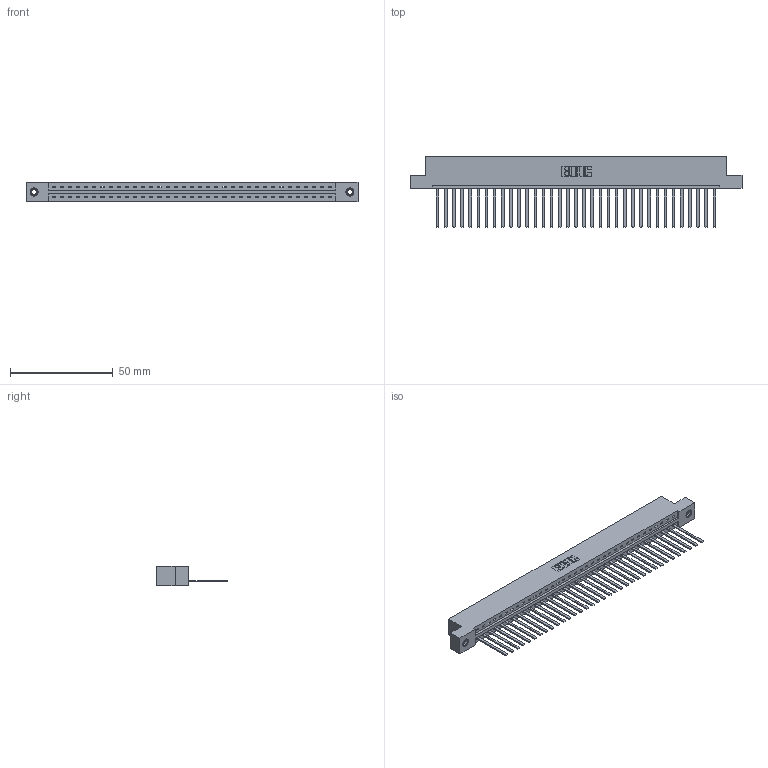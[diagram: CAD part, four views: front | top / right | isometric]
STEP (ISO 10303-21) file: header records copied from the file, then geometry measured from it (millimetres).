
FILE_DESCRIPTION (( 'STEP AP203' ), '1' );
FILE_NAME ('387-035-544-107.STEP', '2018-09-18T22:42:55', ( '' ), ( '' ), 'SwSTEP 2.0', 'SolidWorks 2016', '' );
FILE_SCHEMA (( 'CONFIG_CONTROL_DESIGN' ));
Length unit declared in the file: inch
Products named in the file (4): 337 Part_Flush Mounting Lugs - 0.156 Dia-TI; 345-292-001_345-293-144; 345-250-001_345-250-005-103; 387-035-544-107
Assembly tree (38 placements, depth 2):
  387-035-544-107
    337 Part_Flush Mounting Lugs - 0.156 Dia-TI
    345-292-001_345-293-144  x35
    345-250-001_345-250-005-103  x2
Bounding box: 161.7 x 34.3 x 9.4 mm (x, y, z)
Volume: 17109.9 mm3; surface area: 19016.1 mm2
Topology: 38 solids, 38 shells, 2134 faces, 6397 edges, 4210 vertices
Faces by surface type: plane 1572, cylinder 546, cone 12, torus 4
Entity records: 27924 total; most frequent: CARTESIAN_POINT 4842, ORIENTED_EDGE 4806, DIRECTION 4119, EDGE_CURVE 2403, VECTOR 2259, LINE 2259, VERTEX_POINT 1596, AXIS2_PLACEMENT_3D 930
